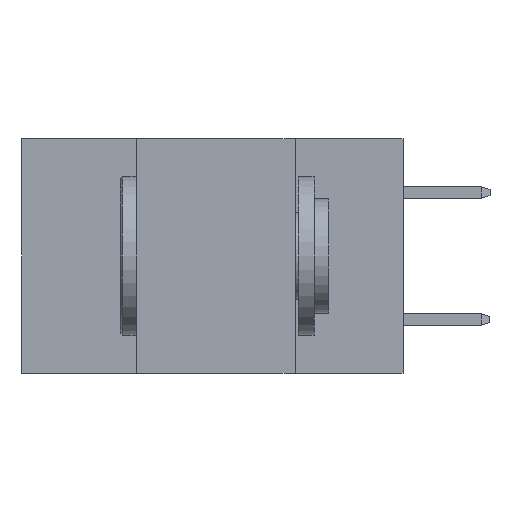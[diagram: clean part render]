
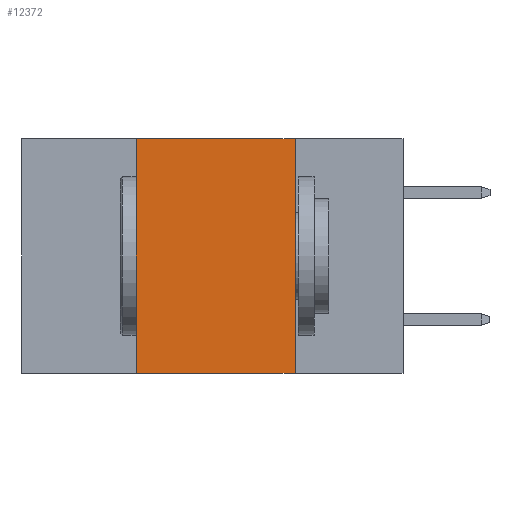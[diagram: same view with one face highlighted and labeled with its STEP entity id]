
A CAD part, left-side view. The second image highlights one B-rep face of the part: STEP entity #12372.
In plain terms, the highlighted planar face has unit normal (-1, 0, 0).
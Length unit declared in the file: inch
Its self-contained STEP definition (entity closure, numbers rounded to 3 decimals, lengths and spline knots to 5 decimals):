
#135 = EDGE_CURVE ( 'NONE', #4801, #11144, #12368, .T. ) ;
#358 = FACE_OUTER_BOUND ( 'NONE', #1869, .T. ) ;
#859 = ORIENTED_EDGE ( 'NONE', *, *, #6924, .F. ) ;
#1579 = ORIENTED_EDGE ( 'NONE', *, *, #135, .F. ) ;
#1869 = EDGE_LOOP ( 'NONE', ( #4261, #1579, #859, #5078 ) ) ;
#2246 = LINE ( 'NONE', #7995, #6263 ) ;
#2265 = CARTESIAN_POINT ( 'NONE',  ( 0., 0.17, -0.37 ) ) ;
#2562 = VECTOR ( 'NONE', #7691, 39.37008 ) ;
#2812 = DIRECTION ( 'NONE',  ( 0., 0., -1. ) ) ;
#3150 = DIRECTION ( 'NONE',  ( 1., 0., 0. ) ) ;
#4208 = AXIS2_PLACEMENT_3D ( 'NONE', #11825, #3150, #10008 ) ;
#4261 = ORIENTED_EDGE ( 'NONE', *, *, #6208, .F. ) ;
#4801 = VERTEX_POINT ( 'NONE', #6217 ) ;
#4895 = CARTESIAN_POINT ( 'NONE',  ( 0., 0.6, -0.37 ) ) ;
#5027 = CARTESIAN_POINT ( 'NONE',  ( 0., 0.17, 0. ) ) ;
#5078 = ORIENTED_EDGE ( 'NONE', *, *, #5080, .T. ) ;
#5080 = EDGE_CURVE ( 'NONE', #10093, #12326, #11611, .T. ) ;
#5531 = CARTESIAN_POINT ( 'NONE',  ( 0., 0.6, 0. ) ) ;
#5895 = LINE ( 'NONE', #11431, #9148 ) ;
#6208 = EDGE_CURVE ( 'NONE', #11144, #12326, #5895, .T. ) ;
#6217 = CARTESIAN_POINT ( 'NONE',  ( 0., 0.42, 0. ) ) ;
#6263 = VECTOR ( 'NONE', #10613, 39.37008 ) ;
#6924 = EDGE_CURVE ( 'NONE', #10093, #4801, #2246, .T. ) ;
#7203 = PLANE ( 'NONE',  #4208 ) ;
#7691 = DIRECTION ( 'NONE',  ( 0., -1., 0. ) ) ;
#7756 = VECTOR ( 'NONE', #12365, 39.37008 ) ;
#7995 = CARTESIAN_POINT ( 'NONE',  ( 0., 0.42, 0. ) ) ;
#9148 = VECTOR ( 'NONE', #2812, 39.37008 ) ;
#9806 = CARTESIAN_POINT ( 'NONE',  ( 0., 0.42, -0.37 ) ) ;
#10008 = DIRECTION ( 'NONE',  ( 0., 0., -1. ) ) ;
#10093 = VERTEX_POINT ( 'NONE', #9806 ) ;
#10613 = DIRECTION ( 'NONE',  ( 0., 0., 1. ) ) ;
#11144 = VERTEX_POINT ( 'NONE', #5027 ) ;
#11431 = CARTESIAN_POINT ( 'NONE',  ( 0., 0.17, 0. ) ) ;
#11611 = LINE ( 'NONE', #4895, #7756 ) ;
#11825 = CARTESIAN_POINT ( 'NONE',  ( 0., 0.6, 0. ) ) ;
#12326 = VERTEX_POINT ( 'NONE', #2265 ) ;
#12365 = DIRECTION ( 'NONE',  ( 0., -1., 0. ) ) ;
#12368 = LINE ( 'NONE', #5531, #2562 ) ;
#12372 = ADVANCED_FACE ( 'NONE', ( #358 ), #7203, .F. ) ;
